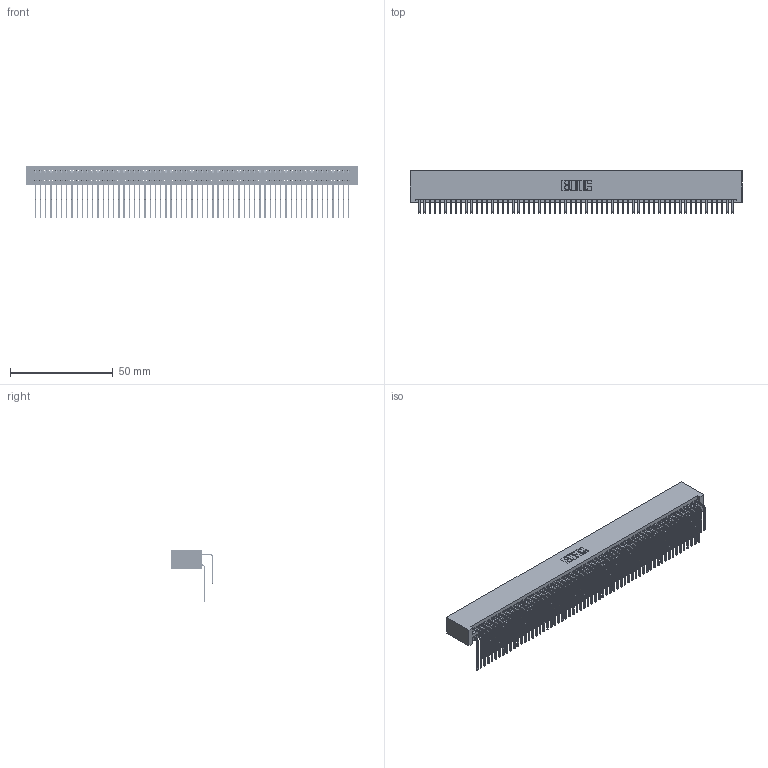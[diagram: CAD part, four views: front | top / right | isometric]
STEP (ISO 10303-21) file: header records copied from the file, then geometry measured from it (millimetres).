
FILE_DESCRIPTION (( 'STEP AP203' ), '1' );
FILE_NAME ('845-122-559-201.STEP', '2018-11-21T14:29:32', ( '' ), ( '' ), 'SwSTEP 2.0', 'SolidWorks 2016', '' );
FILE_SCHEMA (( 'CONFIG_CONTROL_DESIGN' ));
Length unit declared in the file: inch
Products named in the file (4): 345-292-001_558 559 Tail - 1; 345-292-001_559 Tail - 2; 845-122-559-201; 845 Part_No Mounting Lugs
Assembly tree (123 placements, depth 2):
  845-122-559-201
    845 Part_No Mounting Lugs
    345-292-001_558 559 Tail - 1  x61
    345-292-001_559 Tail - 2  x61
Bounding box: 161.54 x 20.56 x 25.53 mm (x, y, z)
Volume: 17188.6 mm3; surface area: 29388.3 mm2
Topology: 123 solids, 123 shells, 6462 faces, 19227 edges, 12654 vertices
Faces by surface type: plane 4346, cylinder 2116
Entity records: 46679 total; most frequent: CARTESIAN_POINT 7851, ORIENTED_EDGE 7734, DIRECTION 6867, EDGE_CURVE 3867, VECTOR 3459, LINE 3459, VERTEX_POINT 2574, AXIS2_PLACEMENT_3D 1704
